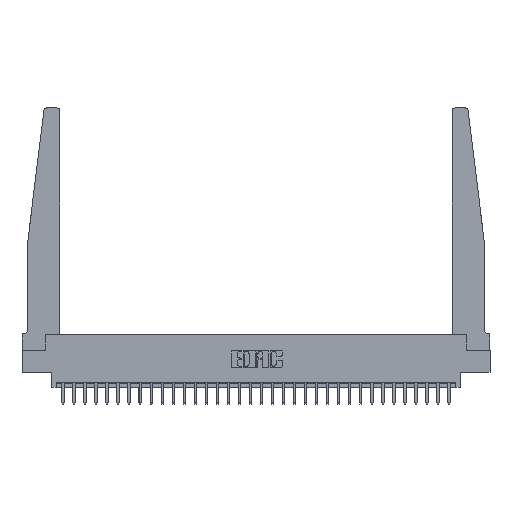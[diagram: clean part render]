
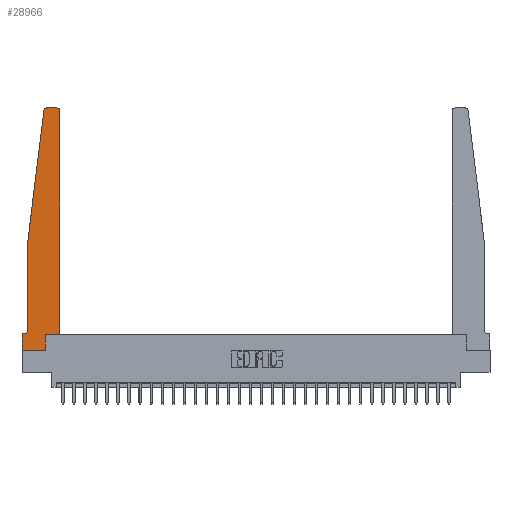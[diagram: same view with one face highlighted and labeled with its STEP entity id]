
A CAD part, top view. The second image highlights one B-rep face of the part: STEP entity #28966.
In plain terms, the highlighted planar face has unit normal (0, 0, 1).
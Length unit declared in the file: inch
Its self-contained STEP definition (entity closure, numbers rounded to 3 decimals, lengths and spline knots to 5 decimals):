
#143 = VECTOR ( 'NONE', #20405, 39.37008 ) ;
#748 = EDGE_CURVE ( 'NONE', #4604, #24645, #18497, .T. ) ;
#911 = CARTESIAN_POINT ( 'NONE',  ( 0.425, 0.18, 0.37 ) ) ;
#1078 = EDGE_CURVE ( 'NONE', #24520, #14578, #11575, .T. ) ;
#1194 = CIRCLE ( 'NONE', #18020, 0.03 ) ;
#1351 = ORIENTED_EDGE ( 'NONE', *, *, #19254, .T. ) ;
#1583 = CARTESIAN_POINT ( 'NONE',  ( 0.065, 1.25, 0.37 ) ) ;
#1590 = AXIS2_PLACEMENT_3D ( 'NONE', #4934, #23028, #2390 ) ;
#1776 = DIRECTION ( 'NONE',  ( 1., 0., 0. ) ) ;
#1840 = VECTOR ( 'NONE', #29170, 39.37008 ) ;
#2166 = VERTEX_POINT ( 'NONE', #24832 ) ;
#2390 = DIRECTION ( 'NONE',  ( 1., 0., 0. ) ) ;
#2409 = LINE ( 'NONE', #4814, #25302 ) ;
#2667 = EDGE_CURVE ( 'NONE', #9719, #4604, #27212, .T. ) ;
#2675 = VECTOR ( 'NONE', #27727, 39.37008 ) ;
#3105 = EDGE_CURVE ( 'NONE', #23489, #29261, #22795, .T. ) ;
#4223 = CARTESIAN_POINT ( 'NONE',  ( 0.425, 0.18, 0.37 ) ) ;
#4234 = CARTESIAN_POINT ( 'NONE',  ( 0.395, 2.72, 0.37 ) ) ;
#4604 = VERTEX_POINT ( 'NONE', #10111 ) ;
#4814 = CARTESIAN_POINT ( 'NONE',  ( 0.2605, 0.18, 0.37 ) ) ;
#4934 = CARTESIAN_POINT ( 'NONE',  ( 0., 0.1875, 0.37 ) ) ;
#4988 = AXIS2_PLACEMENT_3D ( 'NONE', #17254, #19488, #22093 ) ;
#5894 = VERTEX_POINT ( 'NONE', #24906 ) ;
#6411 = LINE ( 'NONE', #911, #23957 ) ;
#6668 = DIRECTION ( 'NONE',  ( 0., -1., 0. ) ) ;
#7287 = VERTEX_POINT ( 'NONE', #20990 ) ;
#7524 = ORIENTED_EDGE ( 'NONE', *, *, #14495, .T. ) ;
#7677 = AXIS2_PLACEMENT_3D ( 'NONE', #8315, #24452, #8177 ) ;
#7996 = VERTEX_POINT ( 'NONE', #12527 ) ;
#8177 = DIRECTION ( 'NONE',  ( 1., 0., 0. ) ) ;
#8315 = CARTESIAN_POINT ( 'NONE',  ( 0.27653, 2.72, 0.37 ) ) ;
#9166 = EDGE_CURVE ( 'NONE', #2166, #9719, #20650, .T. ) ;
#9300 = VERTEX_POINT ( 'NONE', #24596 ) ;
#9581 = CARTESIAN_POINT ( 'NONE',  ( 0.425, 2.72, 0.37 ) ) ;
#9646 = EDGE_LOOP ( 'NONE', ( #29754, #15406, #26876, #10888, #18751, #7524, #14666, #21371, #13305, #1351, #28874, #13902 ) ) ;
#9719 = VERTEX_POINT ( 'NONE', #12787 ) ;
#9930 = FACE_OUTER_BOUND ( 'NONE', #9646, .T. ) ;
#10111 = CARTESIAN_POINT ( 'NONE',  ( 0.065, 1.25, 0.37 ) ) ;
#10119 = EDGE_CURVE ( 'NONE', #24645, #7996, #26182, .T. ) ;
#10888 = ORIENTED_EDGE ( 'NONE', *, *, #748, .T. ) ;
#10981 = LINE ( 'NONE', #29210, #21877 ) ;
#11546 = CARTESIAN_POINT ( 'NONE',  ( 0.2605, 0., 0.37 ) ) ;
#11575 = LINE ( 'NONE', #22862, #17094 ) ;
#12158 = EDGE_CURVE ( 'NONE', #29261, #5894, #2409, .T. ) ;
#12527 = CARTESIAN_POINT ( 'NONE',  ( 0.015, 0.1875, 0.37 ) ) ;
#12787 = CARTESIAN_POINT ( 'NONE',  ( 0.24675, 2.72367, 0.37 ) ) ;
#13305 = ORIENTED_EDGE ( 'NONE', *, *, #12158, .T. ) ;
#13453 = DIRECTION ( 'NONE',  ( 1., 0., 0. ) ) ;
#13832 = PLANE ( 'NONE',  #1590 ) ;
#13859 = CARTESIAN_POINT ( 'NONE',  ( 0.065, 1.25, 0.37 ) ) ;
#13866 = CARTESIAN_POINT ( 'NONE',  ( 0.065, 0.2375, 0.37 ) ) ;
#13902 = ORIENTED_EDGE ( 'NONE', *, *, #15167, .T. ) ;
#13945 = CARTESIAN_POINT ( 'NONE',  ( 0.065, 0.1875, 0.37 ) ) ;
#14495 = EDGE_CURVE ( 'NONE', #7996, #9300, #27059, .T. ) ;
#14578 = VERTEX_POINT ( 'NONE', #9581 ) ;
#14666 = ORIENTED_EDGE ( 'NONE', *, *, #27370, .T. ) ;
#15167 = EDGE_CURVE ( 'NONE', #14578, #7287, #1194, .T. ) ;
#15406 = ORIENTED_EDGE ( 'NONE', *, *, #9166, .T. ) ;
#16152 = CARTESIAN_POINT ( 'NONE',  ( 0., 0., 0.37 ) ) ;
#17094 = VECTOR ( 'NONE', #27397, 39.37008 ) ;
#17254 = CARTESIAN_POINT ( 'NONE',  ( 0.015, 0.2375, 0.37 ) ) ;
#18020 = AXIS2_PLACEMENT_3D ( 'NONE', #4234, #22309, #20178 ) ;
#18497 = LINE ( 'NONE', #13859, #2675 ) ;
#18751 = ORIENTED_EDGE ( 'NONE', *, *, #10119, .T. ) ;
#18845 = CARTESIAN_POINT ( 'NONE',  ( 0., 0., 0.37 ) ) ;
#19254 = EDGE_CURVE ( 'NONE', #5894, #24520, #6411, .T. ) ;
#19488 = DIRECTION ( 'NONE',  ( 0., 0., -1. ) ) ;
#20178 = DIRECTION ( 'NONE',  ( 1., 0., 0. ) ) ;
#20405 = DIRECTION ( 'NONE',  ( -1., 0., 0. ) ) ;
#20650 = CIRCLE ( 'NONE', #7677, 0.03 ) ;
#20940 = EDGE_CURVE ( 'NONE', #7287, #2166, #10981, .T. ) ;
#20990 = CARTESIAN_POINT ( 'NONE',  ( 0.395, 2.75, 0.37 ) ) ;
#21371 = ORIENTED_EDGE ( 'NONE', *, *, #3105, .T. ) ;
#21877 = VECTOR ( 'NONE', #26530, 39.37008 ) ;
#22093 = DIRECTION ( 'NONE',  ( -1., 0., 0. ) ) ;
#22309 = DIRECTION ( 'NONE',  ( 0., 0., 1. ) ) ;
#22795 = LINE ( 'NONE', #16152, #24941 ) ;
#22862 = CARTESIAN_POINT ( 'NONE',  ( 0.425, 0.18, 0.37 ) ) ;
#23028 = DIRECTION ( 'NONE',  ( 0., 0., 1. ) ) ;
#23489 = VERTEX_POINT ( 'NONE', #18845 ) ;
#23957 = VECTOR ( 'NONE', #1776, 39.37008 ) ;
#24452 = DIRECTION ( 'NONE',  ( 0., 0., 1. ) ) ;
#24520 = VERTEX_POINT ( 'NONE', #4223 ) ;
#24596 = CARTESIAN_POINT ( 'NONE',  ( 0., 0.1875, 0.37 ) ) ;
#24633 = VECTOR ( 'NONE', #6668, 39.37008 ) ;
#24645 = VERTEX_POINT ( 'NONE', #13866 ) ;
#24832 = CARTESIAN_POINT ( 'NONE',  ( 0.27653, 2.75, 0.37 ) ) ;
#24906 = CARTESIAN_POINT ( 'NONE',  ( 0.2605, 0.18, 0.37 ) ) ;
#24941 = VECTOR ( 'NONE', #13453, 39.37008 ) ;
#25211 = CARTESIAN_POINT ( 'NONE',  ( 0., 0., 0.37 ) ) ;
#25302 = VECTOR ( 'NONE', #27420, 39.37008 ) ;
#26182 = CIRCLE ( 'NONE', #4988, 0.05 ) ;
#26530 = DIRECTION ( 'NONE',  ( -1., 0., 0. ) ) ;
#26876 = ORIENTED_EDGE ( 'NONE', *, *, #2667, .T. ) ;
#27059 = LINE ( 'NONE', #13945, #143 ) ;
#27212 = LINE ( 'NONE', #1583, #1840 ) ;
#27370 = EDGE_CURVE ( 'NONE', #9300, #23489, #29583, .T. ) ;
#27397 = DIRECTION ( 'NONE',  ( 0., 1., 0. ) ) ;
#27420 = DIRECTION ( 'NONE',  ( 0., 1., 0. ) ) ;
#27727 = DIRECTION ( 'NONE',  ( 0., -1., 0. ) ) ;
#28874 = ORIENTED_EDGE ( 'NONE', *, *, #1078, .T. ) ;
#28966 = ADVANCED_FACE ( 'NONE', ( #9930 ), #13832, .T. ) ;
#29170 = DIRECTION ( 'NONE',  ( -0.122, -0.992, 0. ) ) ;
#29210 = CARTESIAN_POINT ( 'NONE',  ( 0.25, 2.75, 0.37 ) ) ;
#29261 = VERTEX_POINT ( 'NONE', #11546 ) ;
#29583 = LINE ( 'NONE', #25211, #24633 ) ;
#29754 = ORIENTED_EDGE ( 'NONE', *, *, #20940, .T. ) ;
